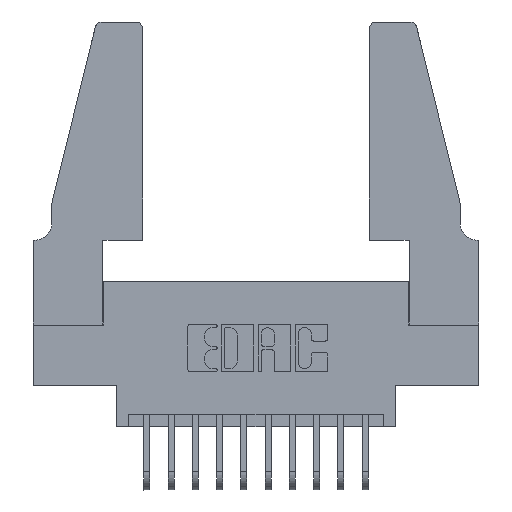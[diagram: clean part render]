
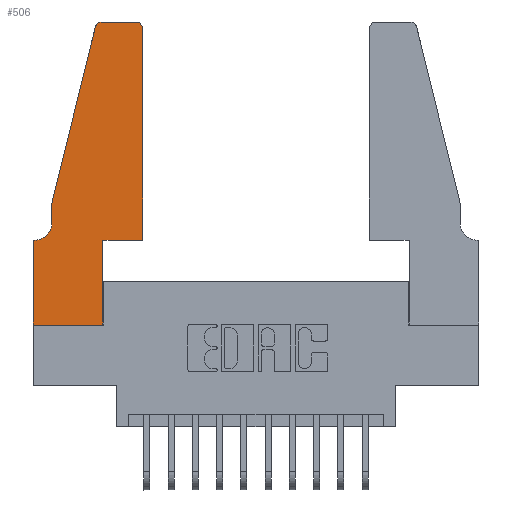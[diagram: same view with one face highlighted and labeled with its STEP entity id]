
A CAD part, top view. The second image highlights one B-rep face of the part: STEP entity #506.
In plain terms, the highlighted planar face has unit normal (0, 0, 1).
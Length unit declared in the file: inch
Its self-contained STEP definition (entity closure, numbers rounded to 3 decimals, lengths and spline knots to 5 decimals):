
#31 = DIRECTION ( 'NONE',  ( 0., 0., -1. ) ) ;
#124 = LINE ( 'NONE', #6021, #11528 ) ;
#283 = CARTESIAN_POINT ( 'NONE',  ( 0.0755, 0.5, 0.37 ) ) ;
#303 = EDGE_CURVE ( 'NONE', #9445, #1235, #3384, .T. ) ;
#441 = DIRECTION ( 'NONE',  ( 0., 1., 0. ) ) ;
#506 = ADVANCED_FACE ( 'NONE', ( #8684 ), #6214, .T. ) ;
#532 = EDGE_CURVE ( 'NONE', #6945, #11942, #14089, .T. ) ;
#932 = ORIENTED_EDGE ( 'NONE', *, *, #12717, .T. ) ;
#1048 = VERTEX_POINT ( 'NONE', #8464 ) ;
#1077 = EDGE_LOOP ( 'NONE', ( #13685, #4336, #3203, #3628, #10895, #932, #3910, #12595, #2065, #5165, #8231, #7629 ) ) ;
#1110 = EDGE_CURVE ( 'NONE', #11942, #2915, #5963, .T. ) ;
#1235 = VERTEX_POINT ( 'NONE', #13650 ) ;
#1275 = VECTOR ( 'NONE', #10211, 39.37008 ) ;
#1365 = CARTESIAN_POINT ( 'NONE',  ( 0., 0., 0.37 ) ) ;
#2027 = CIRCLE ( 'NONE', #8605, 0.03 ) ;
#2065 = ORIENTED_EDGE ( 'NONE', *, *, #3883, .T. ) ;
#2463 = CARTESIAN_POINT ( 'NONE',  ( 0.4505, 0.35, 0.37 ) ) ;
#2915 = VERTEX_POINT ( 'NONE', #10879 ) ;
#2975 = LINE ( 'NONE', #3391, #5920 ) ;
#3010 = EDGE_CURVE ( 'NONE', #1235, #7928, #2975, .T. ) ;
#3137 = DIRECTION ( 'NONE',  ( 0., 0., 1. ) ) ;
#3185 = EDGE_CURVE ( 'NONE', #7928, #3532, #3479, .T. ) ;
#3203 = ORIENTED_EDGE ( 'NONE', *, *, #3010, .T. ) ;
#3384 = CIRCLE ( 'NONE', #10332, 0.03 ) ;
#3391 = CARTESIAN_POINT ( 'NONE',  ( 0.0755, 0.5, 0.37 ) ) ;
#3402 = CARTESIAN_POINT ( 'NONE',  ( 0., 0.35, 0.37 ) ) ;
#3479 = LINE ( 'NONE', #13460, #4166 ) ;
#3532 = VERTEX_POINT ( 'NONE', #5620 ) ;
#3628 = ORIENTED_EDGE ( 'NONE', *, *, #3185, .T. ) ;
#3871 = DIRECTION ( 'NONE',  ( -1., 0., 0. ) ) ;
#3883 = EDGE_CURVE ( 'NONE', #2915, #12974, #8772, .T. ) ;
#3900 = VECTOR ( 'NONE', #9558, 39.37008 ) ;
#3910 = ORIENTED_EDGE ( 'NONE', *, *, #532, .T. ) ;
#4166 = VECTOR ( 'NONE', #5919, 39.37008 ) ;
#4248 = LINE ( 'NONE', #10653, #3900 ) ;
#4336 = ORIENTED_EDGE ( 'NONE', *, *, #303, .T. ) ;
#4698 = DIRECTION ( 'NONE',  ( 1., 0., 0. ) ) ;
#4713 = CARTESIAN_POINT ( 'NONE',  ( 0.284, 1.25, 0.37 ) ) ;
#4987 = CIRCLE ( 'NONE', #11533, 0.07 ) ;
#5115 = CARTESIAN_POINT ( 'NONE',  ( 0.2865, 0.35, 0.37 ) ) ;
#5165 = ORIENTED_EDGE ( 'NONE', *, *, #11929, .T. ) ;
#5467 = VECTOR ( 'NONE', #12801, 39.37008 ) ;
#5620 = CARTESIAN_POINT ( 'NONE',  ( 0.0755, 0.42, 0.37 ) ) ;
#5919 = DIRECTION ( 'NONE',  ( 0., -1., 0. ) ) ;
#5920 = VECTOR ( 'NONE', #12124, 39.37008 ) ;
#5963 = LINE ( 'NONE', #11751, #11063 ) ;
#6021 = CARTESIAN_POINT ( 'NONE',  ( 0.4505, 0.35, 0.37 ) ) ;
#6214 = PLANE ( 'NONE',  #7863 ) ;
#6465 = CARTESIAN_POINT ( 'NONE',  ( 0., 0., 0.37 ) ) ;
#6570 = VECTOR ( 'NONE', #7317, 39.37008 ) ;
#6596 = DIRECTION ( 'NONE',  ( 0., 0., 1. ) ) ;
#6663 = EDGE_CURVE ( 'NONE', #8266, #9445, #4248, .T. ) ;
#6731 = CARTESIAN_POINT ( 'NONE',  ( 0.0055, 0.42, 0.37 ) ) ;
#6945 = VERTEX_POINT ( 'NONE', #3402 ) ;
#7202 = LINE ( 'NONE', #2463, #1275 ) ;
#7317 = DIRECTION ( 'NONE',  ( 0., 1., 0. ) ) ;
#7421 = VERTEX_POINT ( 'NONE', #9504 ) ;
#7629 = ORIENTED_EDGE ( 'NONE', *, *, #11442, .T. ) ;
#7666 = CARTESIAN_POINT ( 'NONE',  ( 0.2865, 0.35, 0.37 ) ) ;
#7833 = DIRECTION ( 'NONE',  ( -1., 0., 0. ) ) ;
#7863 = AXIS2_PLACEMENT_3D ( 'NONE', #7873, #3137, #12609 ) ;
#7873 = CARTESIAN_POINT ( 'NONE',  ( 0., 0.35, 0.37 ) ) ;
#7927 = CARTESIAN_POINT ( 'NONE',  ( 0.284, 1.22, 0.37 ) ) ;
#7928 = VERTEX_POINT ( 'NONE', #283 ) ;
#8231 = ORIENTED_EDGE ( 'NONE', *, *, #10062, .T. ) ;
#8266 = VERTEX_POINT ( 'NONE', #10870 ) ;
#8464 = CARTESIAN_POINT ( 'NONE',  ( 0.4505, 0.35, 0.37 ) ) ;
#8605 = AXIS2_PLACEMENT_3D ( 'NONE', #13062, #6596, #14149 ) ;
#8684 = FACE_OUTER_BOUND ( 'NONE', #1077, .T. ) ;
#8772 = LINE ( 'NONE', #5115, #6570 ) ;
#9445 = VERTEX_POINT ( 'NONE', #4713 ) ;
#9504 = CARTESIAN_POINT ( 'NONE',  ( 0.0055, 0.35, 0.37 ) ) ;
#9558 = DIRECTION ( 'NONE',  ( -1., 0., 0. ) ) ;
#9926 = VERTEX_POINT ( 'NONE', #13348 ) ;
#10062 = EDGE_CURVE ( 'NONE', #1048, #9926, #124, .T. ) ;
#10211 = DIRECTION ( 'NONE',  ( 1., 0., 0. ) ) ;
#10332 = AXIS2_PLACEMENT_3D ( 'NONE', #7927, #13338, #4698 ) ;
#10653 = CARTESIAN_POINT ( 'NONE',  ( 0.2605, 1.25, 0.37 ) ) ;
#10870 = CARTESIAN_POINT ( 'NONE',  ( 0.4205, 1.25, 0.37 ) ) ;
#10879 = CARTESIAN_POINT ( 'NONE',  ( 0.2865, 0., 0.37 ) ) ;
#10895 = ORIENTED_EDGE ( 'NONE', *, *, #11531, .T. ) ;
#11013 = VECTOR ( 'NONE', #3871, 39.37008 ) ;
#11063 = VECTOR ( 'NONE', #12088, 39.37008 ) ;
#11442 = EDGE_CURVE ( 'NONE', #9926, #8266, #2027, .T. ) ;
#11525 = CARTESIAN_POINT ( 'NONE',  ( 0.0755, 0.35, 0.37 ) ) ;
#11528 = VECTOR ( 'NONE', #441, 39.37008 ) ;
#11531 = EDGE_CURVE ( 'NONE', #3532, #7421, #4987, .T. ) ;
#11533 = AXIS2_PLACEMENT_3D ( 'NONE', #6731, #31, #7833 ) ;
#11751 = CARTESIAN_POINT ( 'NONE',  ( 0., 0., 0.37 ) ) ;
#11929 = EDGE_CURVE ( 'NONE', #12974, #1048, #7202, .T. ) ;
#11942 = VERTEX_POINT ( 'NONE', #1365 ) ;
#12088 = DIRECTION ( 'NONE',  ( 1., 0., 0. ) ) ;
#12124 = DIRECTION ( 'NONE',  ( -0.239, -0.971, 0. ) ) ;
#12595 = ORIENTED_EDGE ( 'NONE', *, *, #1110, .T. ) ;
#12609 = DIRECTION ( 'NONE',  ( 1., 0., 0. ) ) ;
#12717 = EDGE_CURVE ( 'NONE', #7421, #6945, #13499, .T. ) ;
#12801 = DIRECTION ( 'NONE',  ( 0., -1., 0. ) ) ;
#12974 = VERTEX_POINT ( 'NONE', #7666 ) ;
#13062 = CARTESIAN_POINT ( 'NONE',  ( 0.4205, 1.22, 0.37 ) ) ;
#13338 = DIRECTION ( 'NONE',  ( 0., 0., 1. ) ) ;
#13348 = CARTESIAN_POINT ( 'NONE',  ( 0.4505, 1.22, 0.37 ) ) ;
#13460 = CARTESIAN_POINT ( 'NONE',  ( 0.0755, 0.5, 0.37 ) ) ;
#13499 = LINE ( 'NONE', #11525, #11013 ) ;
#13650 = CARTESIAN_POINT ( 'NONE',  ( 0.25487, 1.22718, 0.37 ) ) ;
#13685 = ORIENTED_EDGE ( 'NONE', *, *, #6663, .T. ) ;
#14089 = LINE ( 'NONE', #6465, #5467 ) ;
#14149 = DIRECTION ( 'NONE',  ( 1., 0., 0. ) ) ;
